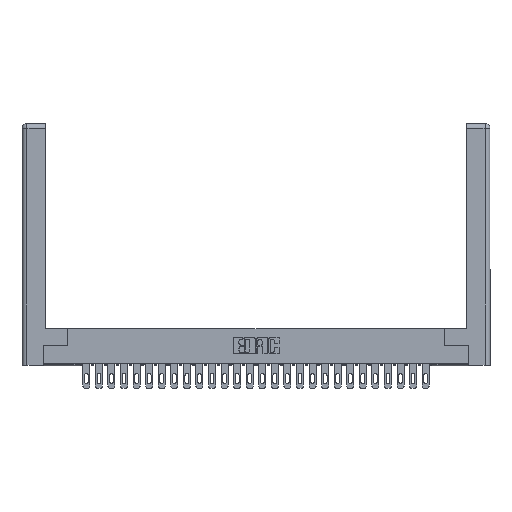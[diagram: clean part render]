
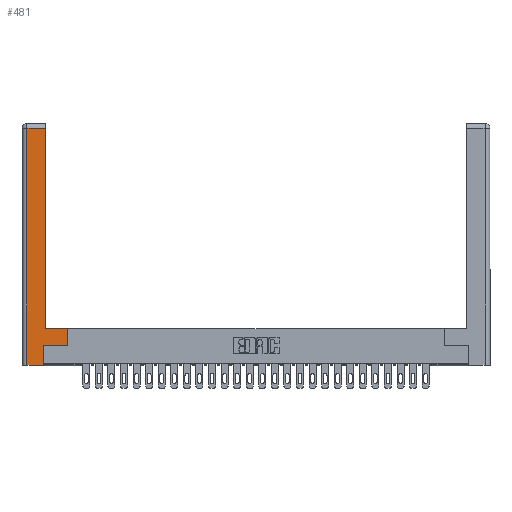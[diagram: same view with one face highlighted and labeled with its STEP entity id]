
A CAD part, top view. The second image highlights one B-rep face of the part: STEP entity #481.
In plain terms, the highlighted planar face has unit normal (0, 0, 1).
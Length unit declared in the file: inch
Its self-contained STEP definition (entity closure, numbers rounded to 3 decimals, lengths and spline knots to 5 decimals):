
#481 = ADVANCED_FACE ( 'NONE', ( #10760 ), #26080, .F. ) ;
#763 = LINE ( 'NONE', #18419, #25370 ) ;
#1572 = DIRECTION ( 'NONE',  ( 1., 0., 0. ) ) ;
#1577 = ORIENTED_EDGE ( 'NONE', *, *, #15436, .T. ) ;
#1650 = LINE ( 'NONE', #20964, #20026 ) ;
#1723 = CARTESIAN_POINT ( 'NONE',  ( 0.565, 0.245, 0. ) ) ;
#2889 = ORIENTED_EDGE ( 'NONE', *, *, #3100, .T. ) ;
#3100 = EDGE_CURVE ( 'NONE', #15576, #28993, #1650, .T. ) ;
#3126 = DIRECTION ( 'NONE',  ( 0., 1., 0. ) ) ;
#4143 = VERTEX_POINT ( 'NONE', #13308 ) ;
#4636 = CARTESIAN_POINT ( 'NONE',  ( 0.0615, 0., 0. ) ) ;
#5848 = EDGE_CURVE ( 'NONE', #19468, #8680, #763, .T. ) ;
#6005 = CARTESIAN_POINT ( 'NONE',  ( 0.265, 0.245, 0. ) ) ;
#6482 = DIRECTION ( 'NONE',  ( 1., 0., 0. ) ) ;
#7520 = DIRECTION ( 'NONE',  ( 0., 0., -1. ) ) ;
#7860 = VECTOR ( 'NONE', #27775, 39.37008 ) ;
#7930 = CARTESIAN_POINT ( 'NONE',  ( 0.295, 3., 0. ) ) ;
#8680 = VERTEX_POINT ( 'NONE', #16371 ) ;
#9152 = DIRECTION ( 'NONE',  ( 0., -1., 0. ) ) ;
#9319 = LINE ( 'NONE', #1723, #27380 ) ;
#9377 = DIRECTION ( 'NONE',  ( -1., 0., 0. ) ) ;
#9976 = ORIENTED_EDGE ( 'NONE', *, *, #5848, .T. ) ;
#10256 = CARTESIAN_POINT ( 'NONE',  ( 0.295, 0.45, 0. ) ) ;
#10433 = ORIENTED_EDGE ( 'NONE', *, *, #21487, .T. ) ;
#10760 = FACE_OUTER_BOUND ( 'NONE', #12103, .T. ) ;
#11113 = VERTEX_POINT ( 'NONE', #15316 ) ;
#12103 = EDGE_LOOP ( 'NONE', ( #17741, #20570, #10433, #2889, #24285, #20292, #9976, #1577 ) ) ;
#12192 = LINE ( 'NONE', #30190, #30136 ) ;
#12221 = CARTESIAN_POINT ( 'NONE',  ( 0.0615, 2.94, 0. ) ) ;
#12362 = EDGE_CURVE ( 'NONE', #28993, #17526, #17077, .T. ) ;
#13308 = CARTESIAN_POINT ( 'NONE',  ( 0.295, 2.94, 0. ) ) ;
#14246 = LINE ( 'NONE', #18413, #7860 ) ;
#15316 = CARTESIAN_POINT ( 'NONE',  ( 0.0615, 2.94, 0. ) ) ;
#15436 = EDGE_CURVE ( 'NONE', #8680, #26226, #14246, .T. ) ;
#15576 = VERTEX_POINT ( 'NONE', #4636 ) ;
#15924 = VECTOR ( 'NONE', #3126, 39.37008 ) ;
#16034 = VECTOR ( 'NONE', #28638, 39.37008 ) ;
#16371 = CARTESIAN_POINT ( 'NONE',  ( 0.565, 0.45, 0. ) ) ;
#17077 = LINE ( 'NONE', #6005, #28770 ) ;
#17526 = VERTEX_POINT ( 'NONE', #21128 ) ;
#17741 = ORIENTED_EDGE ( 'NONE', *, *, #28402, .T. ) ;
#17758 = DIRECTION ( 'NONE',  ( 0., 1., 0. ) ) ;
#18413 = CARTESIAN_POINT ( 'NONE',  ( 0.295, 0.45, 0. ) ) ;
#18419 = CARTESIAN_POINT ( 'NONE',  ( 0.565, 0.45, 0. ) ) ;
#19468 = VERTEX_POINT ( 'NONE', #24984 ) ;
#20026 = VECTOR ( 'NONE', #1572, 39.37008 ) ;
#20292 = ORIENTED_EDGE ( 'NONE', *, *, #25274, .T. ) ;
#20570 = ORIENTED_EDGE ( 'NONE', *, *, #26108, .T. ) ;
#20964 = CARTESIAN_POINT ( 'NONE',  ( 0.265, 0., 0. ) ) ;
#21128 = CARTESIAN_POINT ( 'NONE',  ( 0.265, 0.245, 0. ) ) ;
#21487 = EDGE_CURVE ( 'NONE', #11113, #15576, #12192, .T. ) ;
#22133 = CARTESIAN_POINT ( 'NONE',  ( 0.265, 0., 0. ) ) ;
#23760 = AXIS2_PLACEMENT_3D ( 'NONE', #26124, #7520, #9377 ) ;
#24285 = ORIENTED_EDGE ( 'NONE', *, *, #12362, .T. ) ;
#24984 = CARTESIAN_POINT ( 'NONE',  ( 0.565, 0.245, 0. ) ) ;
#25110 = DIRECTION ( 'NONE',  ( 0., 1., 0. ) ) ;
#25274 = EDGE_CURVE ( 'NONE', #17526, #19468, #9319, .T. ) ;
#25370 = VECTOR ( 'NONE', #17758, 39.37008 ) ;
#26080 = PLANE ( 'NONE',  #23760 ) ;
#26108 = EDGE_CURVE ( 'NONE', #4143, #11113, #28454, .T. ) ;
#26124 = CARTESIAN_POINT ( 'NONE',  ( 0., 0., 0. ) ) ;
#26226 = VERTEX_POINT ( 'NONE', #10256 ) ;
#27380 = VECTOR ( 'NONE', #6482, 39.37008 ) ;
#27775 = DIRECTION ( 'NONE',  ( -1., 0., 0. ) ) ;
#28402 = EDGE_CURVE ( 'NONE', #26226, #4143, #29770, .T. ) ;
#28454 = LINE ( 'NONE', #12221, #16034 ) ;
#28638 = DIRECTION ( 'NONE',  ( -1., 0., 0. ) ) ;
#28770 = VECTOR ( 'NONE', #25110, 39.37008 ) ;
#28993 = VERTEX_POINT ( 'NONE', #22133 ) ;
#29770 = LINE ( 'NONE', #7930, #15924 ) ;
#30136 = VECTOR ( 'NONE', #9152, 39.37008 ) ;
#30190 = CARTESIAN_POINT ( 'NONE',  ( 0.0615, 0., 0. ) ) ;
